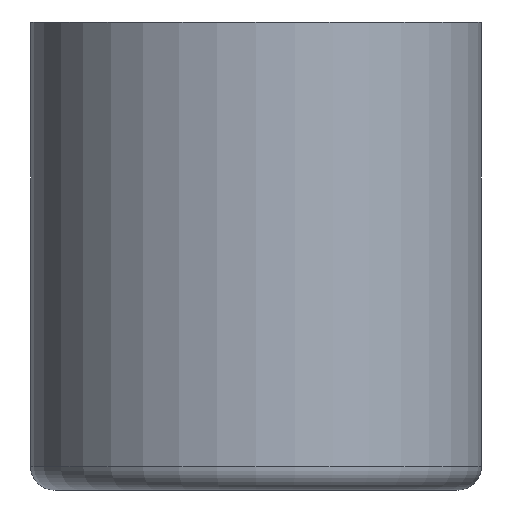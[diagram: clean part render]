
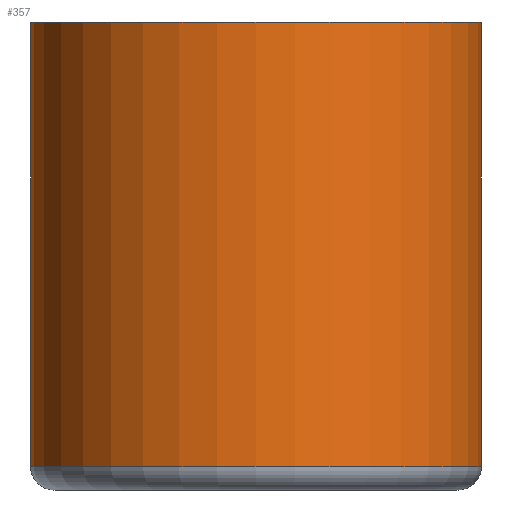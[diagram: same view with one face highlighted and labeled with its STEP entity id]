
A CAD part, front view. The second image highlights one B-rep face of the part: STEP entity #357.
In plain terms, the highlighted cylindrical face has radius 18.352 mm (diameter 36.703 mm), a partial arc.
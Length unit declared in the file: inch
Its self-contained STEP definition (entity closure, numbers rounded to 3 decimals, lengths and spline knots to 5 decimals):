
#24 = VERTEX_POINT ( 'NONE', #1870 ) ;
#213 = VERTEX_POINT ( 'NONE', #2479 ) ;
#238 = CARTESIAN_POINT ( 'NONE',  ( 0., 0., 0. ) ) ;
#343 = LINE ( 'NONE', #3562, #978 ) ;
#357 = ADVANCED_FACE ( 'NONE', ( #2348 ), #3983, .T. ) ;
#398 = VECTOR ( 'NONE', #2420, 39.37008 ) ;
#468 = CARTESIAN_POINT ( 'NONE',  ( 0.7225, 0., -0.25 ) ) ;
#661 = VERTEX_POINT ( 'NONE', #759 ) ;
#684 = EDGE_CURVE ( 'NONE', #213, #1735, #3482, .T. ) ;
#759 = CARTESIAN_POINT ( 'NONE',  ( -0.7225, 0., -0.5 ) ) ;
#824 = EDGE_CURVE ( 'NONE', #661, #1735, #2866, .T. ) ;
#873 = DIRECTION ( 'NONE',  ( -1., 0., 0. ) ) ;
#941 = EDGE_LOOP ( 'NONE', ( #1528, #1054, #3030, #2332, #1765, #2068 ) ) ;
#978 = VECTOR ( 'NONE', #2921, 39.37008 ) ;
#1054 = ORIENTED_EDGE ( 'NONE', *, *, #2083, .T. ) ;
#1124 = AXIS2_PLACEMENT_3D ( 'NONE', #238, #1855, #873 ) ;
#1224 = CARTESIAN_POINT ( 'NONE',  ( -0.7225, 0., 0. ) ) ;
#1408 = CARTESIAN_POINT ( 'NONE',  ( 0., 0., 0. ) ) ;
#1528 = ORIENTED_EDGE ( 'NONE', *, *, #2532, .F. ) ;
#1685 = AXIS2_PLACEMENT_3D ( 'NONE', #3841, #1873, #4177 ) ;
#1735 = VERTEX_POINT ( 'NONE', #1224 ) ;
#1745 = DIRECTION ( 'NONE',  ( -1., 0., 0. ) ) ;
#1765 = ORIENTED_EDGE ( 'NONE', *, *, #2448, .T. ) ;
#1855 = DIRECTION ( 'NONE',  ( 0., 0., -1. ) ) ;
#1870 = CARTESIAN_POINT ( 'NONE',  ( 0.7225, 0., -1.425 ) ) ;
#1873 = DIRECTION ( 'NONE',  ( 0., 0., 1. ) ) ;
#1890 = DIRECTION ( 'NONE',  ( 0., 0., -1. ) ) ;
#1976 = VECTOR ( 'NONE', #3194, 39.37008 ) ;
#2068 = ORIENTED_EDGE ( 'NONE', *, *, #2976, .T. ) ;
#2083 = EDGE_CURVE ( 'NONE', #2677, #213, #2916, .T. ) ;
#2190 = CARTESIAN_POINT ( 'NONE',  ( -0.7225, 0., -0.25 ) ) ;
#2325 = CARTESIAN_POINT ( 'NONE',  ( 0.7225, 0., -0.5 ) ) ;
#2332 = ORIENTED_EDGE ( 'NONE', *, *, #824, .F. ) ;
#2348 = FACE_OUTER_BOUND ( 'NONE', #941, .T. ) ;
#2375 = AXIS2_PLACEMENT_3D ( 'NONE', #1408, #3714, #1745 ) ;
#2420 = DIRECTION ( 'NONE',  ( 0., 0., 1. ) ) ;
#2448 = EDGE_CURVE ( 'NONE', #661, #3793, #2964, .T. ) ;
#2479 = CARTESIAN_POINT ( 'NONE',  ( 0.7225, 0., 0. ) ) ;
#2532 = EDGE_CURVE ( 'NONE', #2677, #24, #343, .T. ) ;
#2677 = VERTEX_POINT ( 'NONE', #2325 ) ;
#2802 = CIRCLE ( 'NONE', #1685, 0.7225 ) ;
#2866 = LINE ( 'NONE', #2190, #1976 ) ;
#2916 = LINE ( 'NONE', #468, #398 ) ;
#2921 = DIRECTION ( 'NONE',  ( 0., 0., -1. ) ) ;
#2964 = LINE ( 'NONE', #4201, #3817 ) ;
#2976 = EDGE_CURVE ( 'NONE', #3793, #24, #2802, .T. ) ;
#3030 = ORIENTED_EDGE ( 'NONE', *, *, #684, .T. ) ;
#3194 = DIRECTION ( 'NONE',  ( 0., 0., 1. ) ) ;
#3318 = CARTESIAN_POINT ( 'NONE',  ( -0.7225, 0., -1.425 ) ) ;
#3482 = CIRCLE ( 'NONE', #2375, 0.7225 ) ;
#3562 = CARTESIAN_POINT ( 'NONE',  ( 0.7225, 0., 0. ) ) ;
#3714 = DIRECTION ( 'NONE',  ( 0., 0., -1. ) ) ;
#3793 = VERTEX_POINT ( 'NONE', #3318 ) ;
#3817 = VECTOR ( 'NONE', #1890, 39.37008 ) ;
#3841 = CARTESIAN_POINT ( 'NONE',  ( 0., 0., -1.425 ) ) ;
#3983 = CYLINDRICAL_SURFACE ( 'NONE', #1124, 0.7225 ) ;
#4177 = DIRECTION ( 'NONE',  ( -1., 0., 0. ) ) ;
#4201 = CARTESIAN_POINT ( 'NONE',  ( -0.7225, 0., 0. ) ) ;
